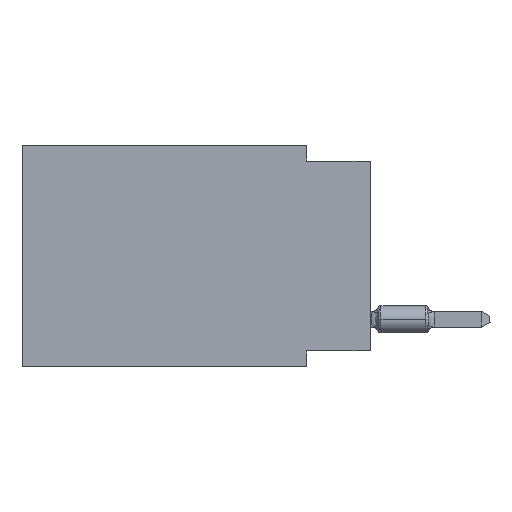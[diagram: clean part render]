
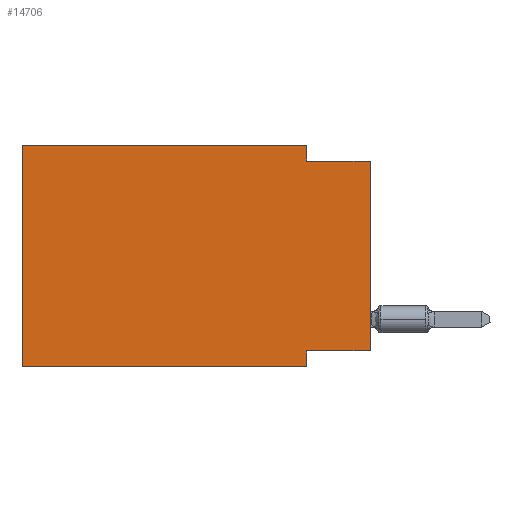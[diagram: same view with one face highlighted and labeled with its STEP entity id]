
A CAD part, left-side view. The second image highlights one B-rep face of the part: STEP entity #14706.
In plain terms, the highlighted planar face has unit normal (-1, 0, 0).
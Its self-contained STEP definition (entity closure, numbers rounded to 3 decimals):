
#282 = CARTESIAN_POINT ( 'NONE',  ( 0., 0., -0.635 ) ) ;
#1095 = CARTESIAN_POINT ( 'NONE',  ( 0., 13.97, 0. ) ) ;
#1210 = CARTESIAN_POINT ( 'NONE',  ( 0., 0., -8.255 ) ) ;
#1408 = ORIENTED_EDGE ( 'NONE', *, *, #44075, .F. ) ;
#1825 = ORIENTED_EDGE ( 'NONE', *, *, #5777, .F. ) ;
#1908 = EDGE_CURVE ( 'NONE', #33716, #11804, #24272, .T. ) ;
#2419 = CARTESIAN_POINT ( 'NONE',  ( 0., 13.97, -8.89 ) ) ;
#2441 = VERTEX_POINT ( 'NONE', #1210 ) ;
#2833 = LINE ( 'NONE', #14087, #22147 ) ;
#4231 = ORIENTED_EDGE ( 'NONE', *, *, #1908, .F. ) ;
#5777 = EDGE_CURVE ( 'NONE', #30852, #33716, #27308, .T. ) ;
#6100 = AXIS2_PLACEMENT_3D ( 'NONE', #13901, #30233, #49688 ) ;
#6480 = FACE_OUTER_BOUND ( 'NONE', #45541, .T. ) ;
#7143 = CARTESIAN_POINT ( 'NONE',  ( 0., 2.54, -8.255 ) ) ;
#7382 = VECTOR ( 'NONE', #48049, 1000. ) ;
#9233 = DIRECTION ( 'NONE',  ( 0., 0., 1. ) ) ;
#10070 = PLANE ( 'NONE',  #6100 ) ;
#11804 = VERTEX_POINT ( 'NONE', #25909 ) ;
#12685 = ORIENTED_EDGE ( 'NONE', *, *, #19307, .F. ) ;
#12794 = VECTOR ( 'NONE', #9233, 1000. ) ;
#13571 = DIRECTION ( 'NONE',  ( 0., -1., 0. ) ) ;
#13901 = CARTESIAN_POINT ( 'NONE',  ( 0., 13.97, 0. ) ) ;
#14087 = CARTESIAN_POINT ( 'NONE',  ( 0., 13.97, -8.89 ) ) ;
#14565 = LINE ( 'NONE', #41659, #43892 ) ;
#14706 = ADVANCED_FACE ( 'NONE', ( #6480 ), #10070, .F. ) ;
#16158 = ORIENTED_EDGE ( 'NONE', *, *, #37461, .F. ) ;
#16894 = CARTESIAN_POINT ( 'NONE',  ( 0., 13.97, 0. ) ) ;
#17802 = EDGE_CURVE ( 'NONE', #2441, #11804, #40514, .T. ) ;
#18413 = DIRECTION ( 'NONE',  ( 0., -1., 0. ) ) ;
#19307 = EDGE_CURVE ( 'NONE', #36273, #29323, #27941, .T. ) ;
#20811 = DIRECTION ( 'NONE',  ( 0., 0., 1. ) ) ;
#22025 = VERTEX_POINT ( 'NONE', #1095 ) ;
#22147 = VECTOR ( 'NONE', #18413, 1000. ) ;
#22569 = CARTESIAN_POINT ( 'NONE',  ( 0., 2.54, 0. ) ) ;
#23596 = CARTESIAN_POINT ( 'NONE',  ( 0., 2.54, -8.89 ) ) ;
#24272 = LINE ( 'NONE', #282, #7382 ) ;
#24659 = VECTOR ( 'NONE', #13571, 1000. ) ;
#25128 = VECTOR ( 'NONE', #20811, 1000. ) ;
#25909 = CARTESIAN_POINT ( 'NONE',  ( 0., 0., -0.635 ) ) ;
#26102 = ORIENTED_EDGE ( 'NONE', *, *, #17802, .T. ) ;
#26203 = CARTESIAN_POINT ( 'NONE',  ( 0., 2.54, -8.89 ) ) ;
#26557 = DIRECTION ( 'NONE',  ( 0., 1., 0. ) ) ;
#27308 = LINE ( 'NONE', #31643, #50282 ) ;
#27495 = EDGE_CURVE ( 'NONE', #2441, #36273, #14565, .T. ) ;
#27941 = LINE ( 'NONE', #23596, #30945 ) ;
#28721 = ORIENTED_EDGE ( 'NONE', *, *, #27495, .F. ) ;
#29323 = VERTEX_POINT ( 'NONE', #26203 ) ;
#30233 = DIRECTION ( 'NONE',  ( 1., 0., 0. ) ) ;
#30852 = VERTEX_POINT ( 'NONE', #22569 ) ;
#30891 = DIRECTION ( 'NONE',  ( 0., 0., -1. ) ) ;
#30945 = VECTOR ( 'NONE', #42776, 1000. ) ;
#31643 = CARTESIAN_POINT ( 'NONE',  ( 0., 2.54, 0. ) ) ;
#33254 = LINE ( 'NONE', #48855, #24659 ) ;
#33349 = CARTESIAN_POINT ( 'NONE',  ( 0., 0., 0. ) ) ;
#33716 = VERTEX_POINT ( 'NONE', #49772 ) ;
#34272 = ORIENTED_EDGE ( 'NONE', *, *, #36351, .T. ) ;
#36273 = VERTEX_POINT ( 'NONE', #7143 ) ;
#36351 = EDGE_CURVE ( 'NONE', #49654, #29323, #2833, .T. ) ;
#37461 = EDGE_CURVE ( 'NONE', #22025, #30852, #33254, .T. ) ;
#39424 = LINE ( 'NONE', #16894, #12794 ) ;
#40514 = LINE ( 'NONE', #33349, #25128 ) ;
#41659 = CARTESIAN_POINT ( 'NONE',  ( 0., 0., -8.255 ) ) ;
#42776 = DIRECTION ( 'NONE',  ( 0., 0., -1. ) ) ;
#43892 = VECTOR ( 'NONE', #26557, 1000. ) ;
#44075 = EDGE_CURVE ( 'NONE', #49654, #22025, #39424, .T. ) ;
#45541 = EDGE_LOOP ( 'NONE', ( #26102, #4231, #1825, #16158, #1408, #34272, #12685, #28721 ) ) ;
#48049 = DIRECTION ( 'NONE',  ( 0., -1., 0. ) ) ;
#48855 = CARTESIAN_POINT ( 'NONE',  ( 0., 13.97, 0. ) ) ;
#49654 = VERTEX_POINT ( 'NONE', #2419 ) ;
#49688 = DIRECTION ( 'NONE',  ( 0., 0., -1. ) ) ;
#49772 = CARTESIAN_POINT ( 'NONE',  ( 0., 2.54, -0.635 ) ) ;
#50282 = VECTOR ( 'NONE', #30891, 1000. ) ;
